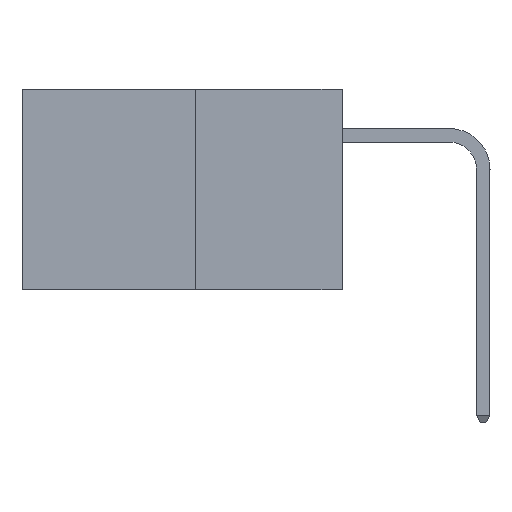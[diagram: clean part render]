
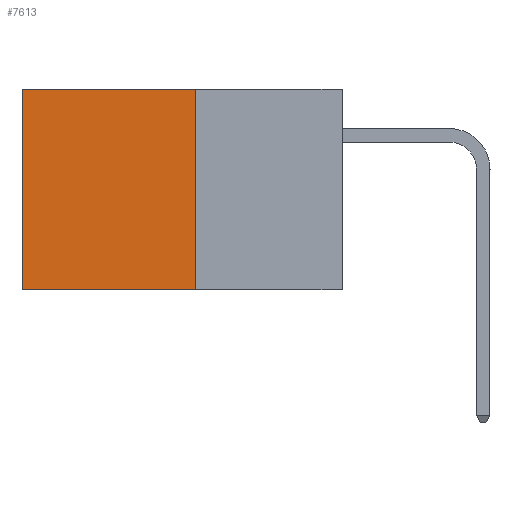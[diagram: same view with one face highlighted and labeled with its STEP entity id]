
A CAD part, left-side view. The second image highlights one B-rep face of the part: STEP entity #7613.
In plain terms, the highlighted planar face has unit normal (-1, 0, 0).
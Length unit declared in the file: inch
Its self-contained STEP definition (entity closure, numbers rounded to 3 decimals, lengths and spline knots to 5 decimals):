
#384 = VERTEX_POINT ( 'NONE', #10941 ) ;
#972 = DIRECTION ( 'NONE',  ( 1., 0., 0. ) ) ;
#1200 = CARTESIAN_POINT ( 'NONE',  ( 0.277, 0.27, -0.37 ) ) ;
#1954 = VERTEX_POINT ( 'NONE', #1200 ) ;
#2746 = AXIS2_PLACEMENT_3D ( 'NONE', #7476, #972, #8521 ) ;
#3154 = PLANE ( 'NONE',  #2746 ) ;
#3261 = CARTESIAN_POINT ( 'NONE',  ( 0.277, 0.27, -0.37 ) ) ;
#4030 = DIRECTION ( 'NONE',  ( 0., 1., 0. ) ) ;
#5175 = CARTESIAN_POINT ( 'NONE',  ( 0.277, 0.59, -0.37 ) ) ;
#5192 = EDGE_CURVE ( 'NONE', #13641, #1954, #10272, .T. ) ;
#5462 = ORIENTED_EDGE ( 'NONE', *, *, #5192, .F. ) ;
#5574 = CARTESIAN_POINT ( 'NONE',  ( 0.277, 0.27, 0. ) ) ;
#5710 = LINE ( 'NONE', #9109, #13684 ) ;
#6204 = CARTESIAN_POINT ( 'NONE',  ( 0.277, 0.27, -0.37 ) ) ;
#7476 = CARTESIAN_POINT ( 'NONE',  ( 0.277, 0.27, -0.37 ) ) ;
#7494 = EDGE_CURVE ( 'NONE', #384, #12483, #13629, .T. ) ;
#7539 = DIRECTION ( 'NONE',  ( 0., 0., -1. ) ) ;
#7613 = ADVANCED_FACE ( 'NONE', ( #12324 ), #3154, .F. ) ;
#8053 = DIRECTION ( 'NONE',  ( 0., 1., 0. ) ) ;
#8144 = VECTOR ( 'NONE', #7539, 39.37008 ) ;
#8348 = ORIENTED_EDGE ( 'NONE', *, *, #7494, .T. ) ;
#8507 = ORIENTED_EDGE ( 'NONE', *, *, #11410, .T. ) ;
#8521 = DIRECTION ( 'NONE',  ( 0., 0., -1. ) ) ;
#9109 = CARTESIAN_POINT ( 'NONE',  ( 0.277, 0.27, 0. ) ) ;
#10007 = EDGE_LOOP ( 'NONE', ( #8348, #12789, #5462, #8507 ) ) ;
#10272 = LINE ( 'NONE', #3261, #8144 ) ;
#10375 = VECTOR ( 'NONE', #4030, 39.37008 ) ;
#10941 = CARTESIAN_POINT ( 'NONE',  ( 0.277, 0.59, 0. ) ) ;
#11410 = EDGE_CURVE ( 'NONE', #13641, #384, #5710, .T. ) ;
#12324 = FACE_OUTER_BOUND ( 'NONE', #10007, .T. ) ;
#12483 = VERTEX_POINT ( 'NONE', #13085 ) ;
#12789 = ORIENTED_EDGE ( 'NONE', *, *, #13389, .F. ) ;
#13085 = CARTESIAN_POINT ( 'NONE',  ( 0.277, 0.59, -0.37 ) ) ;
#13309 = VECTOR ( 'NONE', #13515, 39.37008 ) ;
#13389 = EDGE_CURVE ( 'NONE', #1954, #12483, #13461, .T. ) ;
#13461 = LINE ( 'NONE', #6204, #10375 ) ;
#13515 = DIRECTION ( 'NONE',  ( 0., 0., -1. ) ) ;
#13629 = LINE ( 'NONE', #5175, #13309 ) ;
#13641 = VERTEX_POINT ( 'NONE', #5574 ) ;
#13684 = VECTOR ( 'NONE', #8053, 39.37008 ) ;
